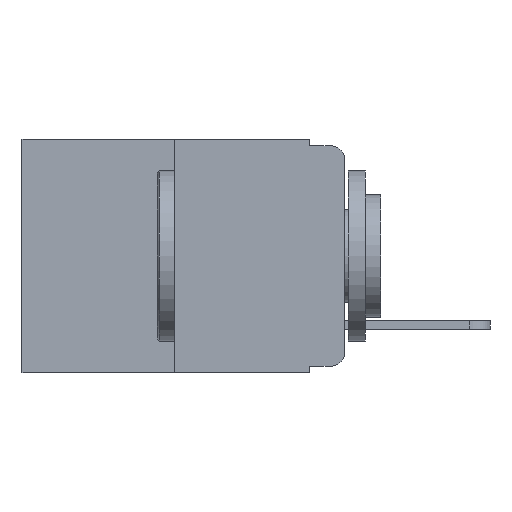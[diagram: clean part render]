
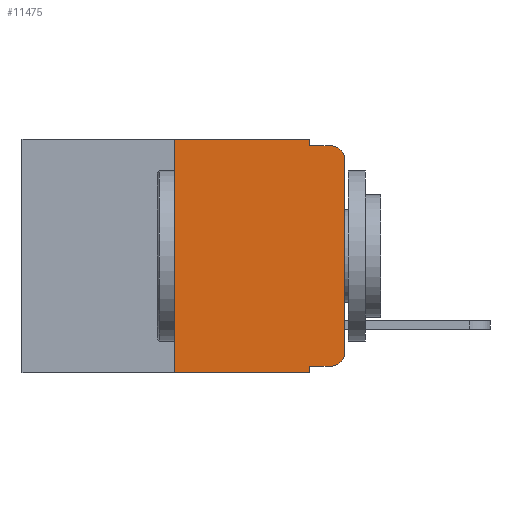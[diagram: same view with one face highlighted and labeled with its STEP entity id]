
A CAD part, left-side view. The second image highlights one B-rep face of the part: STEP entity #11475.
In plain terms, the highlighted planar face has unit normal (-1, 0, 0).
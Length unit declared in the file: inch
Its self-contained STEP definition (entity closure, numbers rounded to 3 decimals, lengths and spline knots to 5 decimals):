
#2 = ORIENTED_EDGE ( 'NONE', *, *, #1066, .F. ) ;
#68 = DIRECTION ( 'NONE',  ( 0., -1., 0. ) ) ;
#180 = ORIENTED_EDGE ( 'NONE', *, *, #1662, .F. ) ;
#254 = VERTEX_POINT ( 'NONE', #3866 ) ;
#271 = ORIENTED_EDGE ( 'NONE', *, *, #10128, .F. ) ;
#290 = VERTEX_POINT ( 'NONE', #6747 ) ;
#385 = ORIENTED_EDGE ( 'NONE', *, *, #1910, .F. ) ;
#497 = CARTESIAN_POINT ( 'NONE',  ( 0., 0.25, 0. ) ) ;
#552 = ORIENTED_EDGE ( 'NONE', *, *, #12037, .T. ) ;
#624 = ORIENTED_EDGE ( 'NONE', *, *, #2167, .F. ) ;
#690 = EDGE_CURVE ( 'NONE', #7445, #4343, #9116, .T. ) ;
#724 = ORIENTED_EDGE ( 'NONE', *, *, #2842, .T. ) ;
#909 = ORIENTED_EDGE ( 'NONE', *, *, #2957, .T. ) ;
#917 = CARTESIAN_POINT ( 'NONE',  ( 0., 0., -0.03 ) ) ;
#929 = EDGE_CURVE ( 'NONE', #4343, #7419, #6601, .T. ) ;
#971 = VERTEX_POINT ( 'NONE', #10828 ) ;
#1066 = EDGE_CURVE ( 'NONE', #290, #7419, #4913, .T. ) ;
#1142 = CARTESIAN_POINT ( 'NONE',  ( 0., 0.25, -0.343 ) ) ;
#1504 = CARTESIAN_POINT ( 'NONE',  ( 0., 0.051, 0. ) ) ;
#1662 = EDGE_CURVE ( 'NONE', #3966, #290, #9431, .T. ) ;
#1816 = CIRCLE ( 'NONE', #2268, 0.02 ) ;
#1910 = EDGE_CURVE ( 'NONE', #5288, #8776, #12170, .T. ) ;
#2011 = VECTOR ( 'NONE', #10948, 39.37008 ) ;
#2167 = EDGE_CURVE ( 'NONE', #2708, #254, #9418, .T. ) ;
#2268 = AXIS2_PLACEMENT_3D ( 'NONE', #9560, #2284, #9382 ) ;
#2284 = DIRECTION ( 'NONE',  ( -1., 0., 0. ) ) ;
#2383 = DIRECTION ( 'NONE',  ( -1., 0., 0. ) ) ;
#2708 = VERTEX_POINT ( 'NONE', #13370 ) ;
#2842 = EDGE_CURVE ( 'NONE', #2708, #971, #11414, .T. ) ;
#2955 = DIRECTION ( 'NONE',  ( 0., -1., 0. ) ) ;
#2957 = EDGE_CURVE ( 'NONE', #971, #7445, #1816, .T. ) ;
#3405 = DIRECTION ( 'NONE',  ( 0., 0., 1. ) ) ;
#3574 = VECTOR ( 'NONE', #9073, 39.37008 ) ;
#3866 = CARTESIAN_POINT ( 'NONE',  ( 0., 0.051, -0.343 ) ) ;
#3966 = VERTEX_POINT ( 'NONE', #10279 ) ;
#4343 = VERTEX_POINT ( 'NONE', #917 ) ;
#4411 = VECTOR ( 'NONE', #3405, 39.37008 ) ;
#4432 = DIRECTION ( 'NONE',  ( 0., 0., -1. ) ) ;
#4558 = FACE_OUTER_BOUND ( 'NONE', #6250, .T. ) ;
#4913 = LINE ( 'NONE', #6829, #12587 ) ;
#5288 = VERTEX_POINT ( 'NONE', #1142 ) ;
#5562 = LINE ( 'NONE', #7432, #10673 ) ;
#6124 = LINE ( 'NONE', #7126, #8464 ) ;
#6250 = EDGE_LOOP ( 'NONE', ( #13028, #10442, #2, #180, #271, #385, #552, #624, #724, #909 ) ) ;
#6601 = CIRCLE ( 'NONE', #8421, 0.02 ) ;
#6747 = CARTESIAN_POINT ( 'NONE',  ( 0., 0.051, -0.01 ) ) ;
#6783 = DIRECTION ( 'NONE',  ( 0., 0., -1. ) ) ;
#6799 = DIRECTION ( 'NONE',  ( 1., 0., 0. ) ) ;
#6829 = CARTESIAN_POINT ( 'NONE',  ( 0., 0.051, -0.01 ) ) ;
#7009 = DIRECTION ( 'NONE',  ( 0., -1., 0. ) ) ;
#7126 = CARTESIAN_POINT ( 'NONE',  ( 0., 0.473, 0. ) ) ;
#7136 = CARTESIAN_POINT ( 'NONE',  ( 0., 0.473, 0. ) ) ;
#7419 = VERTEX_POINT ( 'NONE', #11297 ) ;
#7432 = CARTESIAN_POINT ( 'NONE',  ( 0., 0.473, -0.343 ) ) ;
#7445 = VERTEX_POINT ( 'NONE', #11075 ) ;
#8352 = PLANE ( 'NONE',  #9217 ) ;
#8421 = AXIS2_PLACEMENT_3D ( 'NONE', #8792, #2383, #9834 ) ;
#8464 = VECTOR ( 'NONE', #2955, 39.37008 ) ;
#8776 = VERTEX_POINT ( 'NONE', #497 ) ;
#8792 = CARTESIAN_POINT ( 'NONE',  ( 0., 0.02, -0.03 ) ) ;
#9073 = DIRECTION ( 'NONE',  ( 0., 0., 1. ) ) ;
#9116 = LINE ( 'NONE', #11827, #3574 ) ;
#9217 = AXIS2_PLACEMENT_3D ( 'NONE', #7136, #6799, #6783 ) ;
#9382 = DIRECTION ( 'NONE',  ( 0., 0., -1. ) ) ;
#9418 = LINE ( 'NONE', #1504, #11732 ) ;
#9431 = LINE ( 'NONE', #9590, #12315 ) ;
#9560 = CARTESIAN_POINT ( 'NONE',  ( 0., 0.02, -0.313 ) ) ;
#9590 = CARTESIAN_POINT ( 'NONE',  ( 0., 0.051, 0. ) ) ;
#9834 = DIRECTION ( 'NONE',  ( 0., 0., -1. ) ) ;
#10128 = EDGE_CURVE ( 'NONE', #8776, #3966, #6124, .T. ) ;
#10279 = CARTESIAN_POINT ( 'NONE',  ( 0., 0.051, 0. ) ) ;
#10442 = ORIENTED_EDGE ( 'NONE', *, *, #929, .T. ) ;
#10673 = VECTOR ( 'NONE', #7009, 39.37008 ) ;
#10828 = CARTESIAN_POINT ( 'NONE',  ( 0., 0.02, -0.333 ) ) ;
#10948 = DIRECTION ( 'NONE',  ( 0., -1., 0. ) ) ;
#10971 = CARTESIAN_POINT ( 'NONE',  ( 0., 0.051, -0.333 ) ) ;
#11075 = CARTESIAN_POINT ( 'NONE',  ( 0., 0., -0.313 ) ) ;
#11190 = DIRECTION ( 'NONE',  ( 0., 0., -1. ) ) ;
#11297 = CARTESIAN_POINT ( 'NONE',  ( 0., 0.02, -0.01 ) ) ;
#11351 = CARTESIAN_POINT ( 'NONE',  ( 0., 0.25, 0. ) ) ;
#11414 = LINE ( 'NONE', #10971, #2011 ) ;
#11475 = ADVANCED_FACE ( 'NONE', ( #4558 ), #8352, .F. ) ;
#11732 = VECTOR ( 'NONE', #11190, 39.37008 ) ;
#11827 = CARTESIAN_POINT ( 'NONE',  ( 0., 0., 0. ) ) ;
#12037 = EDGE_CURVE ( 'NONE', #5288, #254, #5562, .T. ) ;
#12170 = LINE ( 'NONE', #11351, #4411 ) ;
#12315 = VECTOR ( 'NONE', #4432, 39.37008 ) ;
#12587 = VECTOR ( 'NONE', #68, 39.37008 ) ;
#13028 = ORIENTED_EDGE ( 'NONE', *, *, #690, .T. ) ;
#13370 = CARTESIAN_POINT ( 'NONE',  ( 0., 0.051, -0.333 ) ) ;
